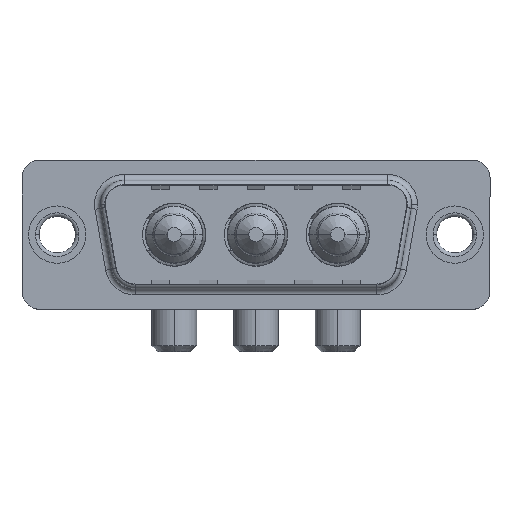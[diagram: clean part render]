
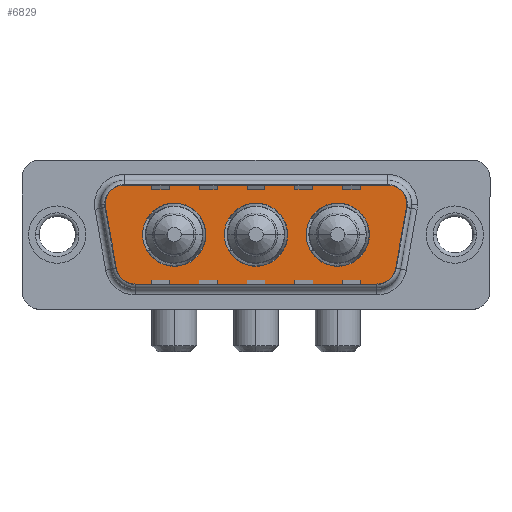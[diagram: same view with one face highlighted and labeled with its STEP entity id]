
A CAD part, top view. The second image highlights one B-rep face of the part: STEP entity #6829.
In plain terms, the highlighted planar face has unit normal (0, 0, 1).
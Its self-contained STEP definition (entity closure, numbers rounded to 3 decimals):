
#54 = EDGE_CURVE ( 'NONE', #8450, #8557, #2022, .T. ) ;
#55 = DIRECTION ( 'NONE',  ( 0.174, -0.985, 0. ) ) ;
#118 = EDGE_CURVE ( 'NONE', #6454, #2103, #10678, .T. ) ;
#152 = DIRECTION ( 'NONE',  ( 0., 0., 1. ) ) ;
#252 = EDGE_CURVE ( 'NONE', #9023, #6211, #7371, .T. ) ;
#273 = LINE ( 'NONE', #7303, #7970 ) ;
#340 = CARTESIAN_POINT ( 'NONE',  ( 6.434, -4.9, 0. ) ) ;
#400 = DIRECTION ( 'NONE',  ( 1., 0., 0. ) ) ;
#533 = CIRCLE ( 'NONE', #6623, 2.65 ) ;
#607 = EDGE_CURVE ( 'NONE', #1036, #10217, #10285, .T. ) ;
#840 = PLANE ( 'NONE',  #10585 ) ;
#952 = CARTESIAN_POINT ( 'NONE',  ( 26.866, -2.9, 0. ) ) ;
#978 = AXIS2_PLACEMENT_3D ( 'NONE', #2093, #9951, #7317 ) ;
#1036 = VERTEX_POINT ( 'NONE', #4180 ) ;
#1064 = ORIENTED_EDGE ( 'NONE', *, *, #4883, .F. ) ;
#1112 = AXIS2_PLACEMENT_3D ( 'NONE', #2863, #9777, #4547 ) ;
#1124 = EDGE_CURVE ( 'NONE', #2944, #4125, #9941, .T. ) ;
#1133 = VECTOR ( 'NONE', #3660, 1000. ) ;
#1321 = DIRECTION ( 'NONE',  ( 1., 0., 0. ) ) ;
#1344 = EDGE_CURVE ( 'NONE', #2588, #8473, #1871, .T. ) ;
#1367 = ORIENTED_EDGE ( 'NONE', *, *, #118, .T. ) ;
#1565 = DIRECTION ( 'NONE',  ( 0., 0., 1. ) ) ;
#1693 = EDGE_CURVE ( 'NONE', #8473, #8450, #273, .T. ) ;
#1871 = CIRCLE ( 'NONE', #978, 2. ) ;
#1954 = VERTEX_POINT ( 'NONE', #3628 ) ;
#2022 = CIRCLE ( 'NONE', #5243, 2. ) ;
#2051 = EDGE_LOOP ( 'NONE', ( #3088, #8209 ) ) ;
#2052 = CARTESIAN_POINT ( 'NONE',  ( 29.859, 2.553, 0. ) ) ;
#2093 = CARTESIAN_POINT ( 'NONE',  ( 27.889, 2.9, 0. ) ) ;
#2103 = VERTEX_POINT ( 'NONE', #10304 ) ;
#2179 = DIRECTION ( 'NONE',  ( 0., 0., 1. ) ) ;
#2294 = CARTESIAN_POINT ( 'NONE',  ( 27.889, 4.9, 0. ) ) ;
#2306 = CARTESIAN_POINT ( 'NONE',  ( 29.859, 2.553, 0. ) ) ;
#2318 = CARTESIAN_POINT ( 'NONE',  ( 19.3, 0., 0. ) ) ;
#2442 = EDGE_CURVE ( 'NONE', #7755, #6454, #4199, .T. ) ;
#2518 = FACE_BOUND ( 'NONE', #4604, .T. ) ;
#2588 = VERTEX_POINT ( 'NONE', #4342 ) ;
#2863 = CARTESIAN_POINT ( 'NONE',  ( 27.889, 2.9, 0. ) ) ;
#2944 = VERTEX_POINT ( 'NONE', #2318 ) ;
#2988 = ORIENTED_EDGE ( 'NONE', *, *, #9834, .F. ) ;
#3087 = CARTESIAN_POINT ( 'NONE',  ( 26.866, -2.9, 0. ) ) ;
#3088 = ORIENTED_EDGE ( 'NONE', *, *, #1124, .F. ) ;
#3120 = AXIS2_PLACEMENT_3D ( 'NONE', #9271, #7353, #5842 ) ;
#3223 = CARTESIAN_POINT ( 'NONE',  ( 16.65, 0., 0. ) ) ;
#3427 = AXIS2_PLACEMENT_3D ( 'NONE', #10992, #9938, #9166 ) ;
#3453 = ORIENTED_EDGE ( 'NONE', *, *, #1344, .T. ) ;
#3522 = EDGE_CURVE ( 'NONE', #4125, #2944, #4071, .T. ) ;
#3628 = CARTESIAN_POINT ( 'NONE',  ( 7.15, 0., 0. ) ) ;
#3660 = DIRECTION ( 'NONE',  ( 1., 0., 0. ) ) ;
#3748 = EDGE_LOOP ( 'NONE', ( #1064, #3766 ) ) ;
#3766 = ORIENTED_EDGE ( 'NONE', *, *, #607, .F. ) ;
#3881 = ORIENTED_EDGE ( 'NONE', *, *, #54, .T. ) ;
#3916 = CIRCLE ( 'NONE', #4097, 2.65 ) ;
#4009 = DIRECTION ( 'NONE',  ( 1., 0., 0. ) ) ;
#4012 = AXIS2_PLACEMENT_3D ( 'NONE', #3087, #1565, #9216 ) ;
#4071 = CIRCLE ( 'NONE', #7302, 2.65 ) ;
#4097 = AXIS2_PLACEMENT_3D ( 'NONE', #9770, #2179, #9819 ) ;
#4119 = ORIENTED_EDGE ( 'NONE', *, *, #252, .T. ) ;
#4125 = VERTEX_POINT ( 'NONE', #7382 ) ;
#4180 = CARTESIAN_POINT ( 'NONE',  ( 20.85, 0., 0. ) ) ;
#4199 = CIRCLE ( 'NONE', #10478, 2. ) ;
#4264 = FACE_BOUND ( 'NONE', #2051, .T. ) ;
#4342 = CARTESIAN_POINT ( 'NONE',  ( 29.889, 2.9, 0. ) ) ;
#4352 = CARTESIAN_POINT ( 'NONE',  ( 28.836, -3.247, 0. ) ) ;
#4375 = FACE_BOUND ( 'NONE', #3748, .T. ) ;
#4455 = VECTOR ( 'NONE', #55, 1000. ) ;
#4547 = DIRECTION ( 'NONE',  ( -1., 0., 0. ) ) ;
#4602 = DIRECTION ( 'NONE',  ( -1., 0., 0. ) ) ;
#4604 = EDGE_LOOP ( 'NONE', ( #2988, #8497 ) ) ;
#4626 = DIRECTION ( 'NONE',  ( 0., 0., 1. ) ) ;
#4667 = CARTESIAN_POINT ( 'NONE',  ( 5.411, 2.9, 0. ) ) ;
#4678 = EDGE_CURVE ( 'NONE', #8557, #7755, #9172, .T. ) ;
#4883 = EDGE_CURVE ( 'NONE', #10217, #1036, #3916, .T. ) ;
#5070 = DIRECTION ( 'NONE',  ( 0., 0., 1. ) ) ;
#5073 = VECTOR ( 'NONE', #10781, 1000. ) ;
#5218 = FACE_OUTER_BOUND ( 'NONE', #6910, .T. ) ;
#5243 = AXIS2_PLACEMENT_3D ( 'NONE', #4667, #8117, #400 ) ;
#5310 = CARTESIAN_POINT ( 'NONE',  ( 26.15, 0., 0. ) ) ;
#5424 = CARTESIAN_POINT ( 'NONE',  ( 9.8, 0., 0. ) ) ;
#5842 = DIRECTION ( 'NONE',  ( 1., 0., 0. ) ) ;
#5952 = CIRCLE ( 'NONE', #1112, 2. ) ;
#6051 = ORIENTED_EDGE ( 'NONE', *, *, #8539, .T. ) ;
#6119 = CARTESIAN_POINT ( 'NONE',  ( 16.65, 0., 0. ) ) ;
#6200 = EDGE_CURVE ( 'NONE', #1954, #6770, #533, .T. ) ;
#6211 = VERTEX_POINT ( 'NONE', #2052 ) ;
#6454 = VERTEX_POINT ( 'NONE', #9452 ) ;
#6623 = AXIS2_PLACEMENT_3D ( 'NONE', #5424, #4626, #1321 ) ;
#6656 = DIRECTION ( 'NONE',  ( 0., 0., 1. ) ) ;
#6744 = DIRECTION ( 'NONE',  ( 0., 0., 1. ) ) ;
#6770 = VERTEX_POINT ( 'NONE', #10061 ) ;
#6829 = ADVANCED_FACE ( 'NONE', ( #4264, #4375, #2518, #5218 ), #840, .T. ) ;
#6910 = EDGE_LOOP ( 'NONE', ( #6051, #4119, #10315, #3453, #9962, #3881, #7624, #9705, #1367 ) ) ;
#7302 = AXIS2_PLACEMENT_3D ( 'NONE', #6119, #152, #9432 ) ;
#7303 = CARTESIAN_POINT ( 'NONE',  ( 5.411, 4.9, 0. ) ) ;
#7317 = DIRECTION ( 'NONE',  ( -1., 0., 0. ) ) ;
#7353 = DIRECTION ( 'NONE',  ( 0., 0., 1. ) ) ;
#7371 = LINE ( 'NONE', #2306, #5073 ) ;
#7382 = CARTESIAN_POINT ( 'NONE',  ( 14., 0., 0. ) ) ;
#7438 = AXIS2_PLACEMENT_3D ( 'NONE', #3223, #6656, #4009 ) ;
#7624 = ORIENTED_EDGE ( 'NONE', *, *, #4678, .T. ) ;
#7671 = CARTESIAN_POINT ( 'NONE',  ( 6.434, -2.9, 0. ) ) ;
#7755 = VERTEX_POINT ( 'NONE', #7835 ) ;
#7835 = CARTESIAN_POINT ( 'NONE',  ( 4.464, -3.247, 0. ) ) ;
#7970 = VECTOR ( 'NONE', #4602, 1000. ) ;
#8117 = DIRECTION ( 'NONE',  ( 0., 0., 1. ) ) ;
#8209 = ORIENTED_EDGE ( 'NONE', *, *, #3522, .F. ) ;
#8295 = CIRCLE ( 'NONE', #3427, 2.65 ) ;
#8377 = EDGE_CURVE ( 'NONE', #6211, #2588, #5952, .T. ) ;
#8410 = DIRECTION ( 'NONE',  ( -1., 0., 0. ) ) ;
#8450 = VERTEX_POINT ( 'NONE', #9986 ) ;
#8473 = VERTEX_POINT ( 'NONE', #2294 ) ;
#8497 = ORIENTED_EDGE ( 'NONE', *, *, #6200, .F. ) ;
#8539 = EDGE_CURVE ( 'NONE', #2103, #9023, #9050, .T. ) ;
#8557 = VERTEX_POINT ( 'NONE', #9051 ) ;
#9023 = VERTEX_POINT ( 'NONE', #4352 ) ;
#9050 = CIRCLE ( 'NONE', #4012, 2. ) ;
#9051 = CARTESIAN_POINT ( 'NONE',  ( 3.441, 2.553, 0. ) ) ;
#9166 = DIRECTION ( 'NONE',  ( 1., 0., 0. ) ) ;
#9172 = LINE ( 'NONE', #10321, #4455 ) ;
#9216 = DIRECTION ( 'NONE',  ( 1., 0., 0. ) ) ;
#9271 = CARTESIAN_POINT ( 'NONE',  ( 23.5, 0., 0. ) ) ;
#9432 = DIRECTION ( 'NONE',  ( 1., 0., 0. ) ) ;
#9452 = CARTESIAN_POINT ( 'NONE',  ( 6.434, -4.9, 0. ) ) ;
#9705 = ORIENTED_EDGE ( 'NONE', *, *, #2442, .T. ) ;
#9770 = CARTESIAN_POINT ( 'NONE',  ( 23.5, 0., 0. ) ) ;
#9777 = DIRECTION ( 'NONE',  ( 0., 0., 1. ) ) ;
#9819 = DIRECTION ( 'NONE',  ( 1., 0., 0. ) ) ;
#9834 = EDGE_CURVE ( 'NONE', #6770, #1954, #8295, .T. ) ;
#9938 = DIRECTION ( 'NONE',  ( 0., 0., 1. ) ) ;
#9941 = CIRCLE ( 'NONE', #7438, 2.65 ) ;
#9951 = DIRECTION ( 'NONE',  ( 0., 0., 1. ) ) ;
#9962 = ORIENTED_EDGE ( 'NONE', *, *, #1693, .T. ) ;
#9986 = CARTESIAN_POINT ( 'NONE',  ( 5.411, 4.9, 0. ) ) ;
#10061 = CARTESIAN_POINT ( 'NONE',  ( 12.45, 0., 0. ) ) ;
#10217 = VERTEX_POINT ( 'NONE', #5310 ) ;
#10267 = DIRECTION ( 'NONE',  ( 1., 0., 0. ) ) ;
#10285 = CIRCLE ( 'NONE', #3120, 2.65 ) ;
#10304 = CARTESIAN_POINT ( 'NONE',  ( 26.866, -4.9, 0. ) ) ;
#10315 = ORIENTED_EDGE ( 'NONE', *, *, #8377, .T. ) ;
#10321 = CARTESIAN_POINT ( 'NONE',  ( 3.441, 2.553, 0. ) ) ;
#10478 = AXIS2_PLACEMENT_3D ( 'NONE', #7671, #5070, #8410 ) ;
#10585 = AXIS2_PLACEMENT_3D ( 'NONE', #952, #6744, #10267 ) ;
#10678 = LINE ( 'NONE', #340, #1133 ) ;
#10781 = DIRECTION ( 'NONE',  ( 0.174, 0.985, 0. ) ) ;
#10992 = CARTESIAN_POINT ( 'NONE',  ( 9.8, 0., 0. ) ) ;
